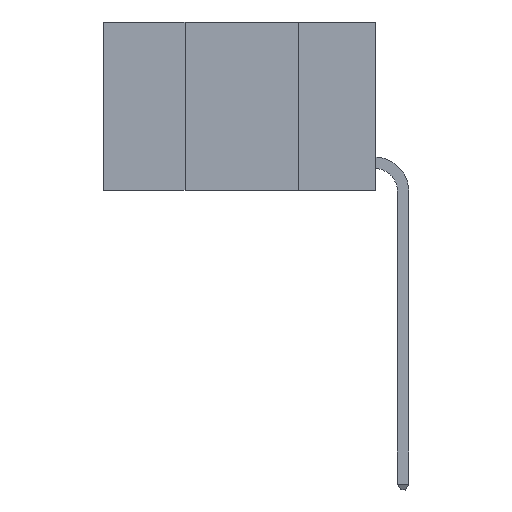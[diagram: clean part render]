
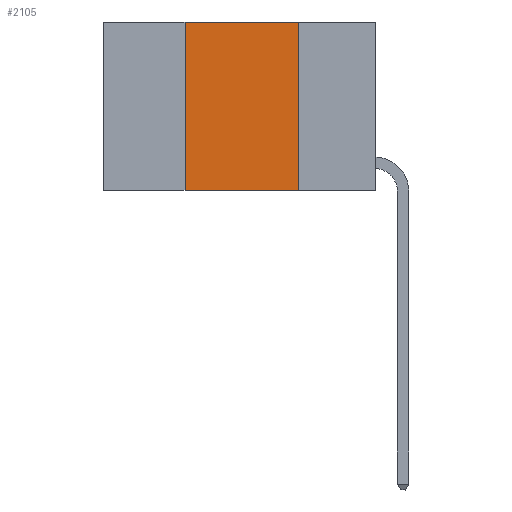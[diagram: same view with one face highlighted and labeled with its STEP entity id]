
A CAD part, left-side view. The second image highlights one B-rep face of the part: STEP entity #2105.
In plain terms, the highlighted planar face has unit normal (-1, 0, 0).
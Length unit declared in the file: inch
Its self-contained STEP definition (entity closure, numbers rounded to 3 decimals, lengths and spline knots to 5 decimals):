
#222 = ORIENTED_EDGE ( 'NONE', *, *, #4015, .F. ) ;
#2105 = ADVANCED_FACE ( 'NONE', ( #6681 ), #6450, .F. ) ;
#2419 = CARTESIAN_POINT ( 'NONE',  ( 0., 0.6, 0. ) ) ;
#2568 = DIRECTION ( 'NONE',  ( 1., 0., 0. ) ) ;
#2764 = ORIENTED_EDGE ( 'NONE', *, *, #24341, .T. ) ;
#2947 = CARTESIAN_POINT ( 'NONE',  ( 0., 0.42, 0. ) ) ;
#4015 = EDGE_CURVE ( 'NONE', #6565, #8216, #23846, .T. ) ;
#4451 = CARTESIAN_POINT ( 'NONE',  ( 0., 0.42, 0. ) ) ;
#4757 = ORIENTED_EDGE ( 'NONE', *, *, #5370, .F. ) ;
#5370 = EDGE_CURVE ( 'NONE', #19744, #10332, #17680, .T. ) ;
#6221 = EDGE_CURVE ( 'NONE', #8216, #19744, #22834, .T. ) ;
#6437 = DIRECTION ( 'NONE',  ( 0., 0., 1. ) ) ;
#6450 = PLANE ( 'NONE',  #8559 ) ;
#6565 = VERTEX_POINT ( 'NONE', #11384 ) ;
#6681 = FACE_OUTER_BOUND ( 'NONE', #20655, .T. ) ;
#7108 = VECTOR ( 'NONE', #24137, 39.37008 ) ;
#8216 = VERTEX_POINT ( 'NONE', #2947 ) ;
#8559 = AXIS2_PLACEMENT_3D ( 'NONE', #10401, #2568, #16373 ) ;
#9060 = CARTESIAN_POINT ( 'NONE',  ( 0., 0.17, 0. ) ) ;
#10332 = VERTEX_POINT ( 'NONE', #13329 ) ;
#10401 = CARTESIAN_POINT ( 'NONE',  ( 0., 0.6, 0. ) ) ;
#11384 = CARTESIAN_POINT ( 'NONE',  ( 0., 0.42, -0.37 ) ) ;
#12405 = VECTOR ( 'NONE', #15015, 39.37008 ) ;
#13329 = CARTESIAN_POINT ( 'NONE',  ( 0., 0.17, -0.37 ) ) ;
#13364 = VECTOR ( 'NONE', #6437, 39.37008 ) ;
#15015 = DIRECTION ( 'NONE',  ( 0., 0., -1. ) ) ;
#16373 = DIRECTION ( 'NONE',  ( 0., 0., -1. ) ) ;
#17353 = LINE ( 'NONE', #21511, #21913 ) ;
#17680 = LINE ( 'NONE', #9060, #12405 ) ;
#19744 = VERTEX_POINT ( 'NONE', #24272 ) ;
#20655 = EDGE_LOOP ( 'NONE', ( #4757, #21594, #222, #2764 ) ) ;
#21511 = CARTESIAN_POINT ( 'NONE',  ( 0., 0.6, -0.37 ) ) ;
#21582 = DIRECTION ( 'NONE',  ( 0., -1., 0. ) ) ;
#21594 = ORIENTED_EDGE ( 'NONE', *, *, #6221, .F. ) ;
#21913 = VECTOR ( 'NONE', #21582, 39.37008 ) ;
#22834 = LINE ( 'NONE', #2419, #7108 ) ;
#23846 = LINE ( 'NONE', #4451, #13364 ) ;
#24137 = DIRECTION ( 'NONE',  ( 0., -1., 0. ) ) ;
#24272 = CARTESIAN_POINT ( 'NONE',  ( 0., 0.17, 0. ) ) ;
#24341 = EDGE_CURVE ( 'NONE', #6565, #10332, #17353, .T. ) ;
